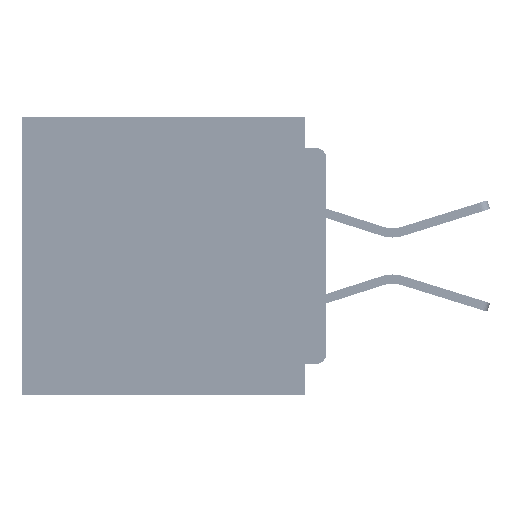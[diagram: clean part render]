
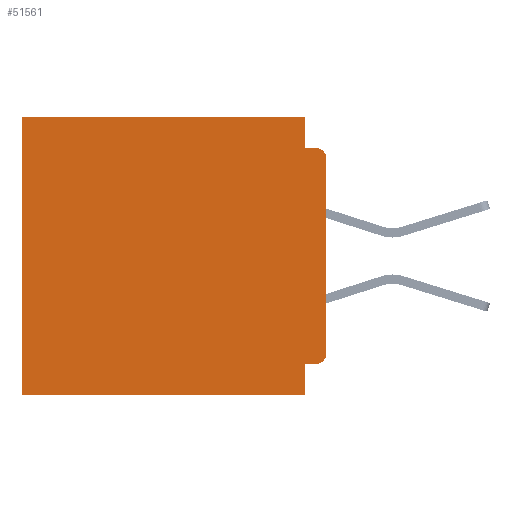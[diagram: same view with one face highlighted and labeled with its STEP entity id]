
A CAD part, left-side view. The second image highlights one B-rep face of the part: STEP entity #51561.
In plain terms, the highlighted planar face has unit normal (-1, 0, 0).
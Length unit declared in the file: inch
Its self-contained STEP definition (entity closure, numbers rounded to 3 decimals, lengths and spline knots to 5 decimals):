
#1955 = ORIENTED_EDGE ( 'NONE', *, *, #10316, .T. ) ;
#1964 = VERTEX_POINT ( 'NONE', #22552 ) ;
#2146 = ORIENTED_EDGE ( 'NONE', *, *, #38919, .F. ) ;
#2992 = CARTESIAN_POINT ( 'NONE',  ( 0.3, 0.031, -0.045 ) ) ;
#3747 = VECTOR ( 'NONE', #14374, 39.37008 ) ;
#8459 = LINE ( 'NONE', #29916, #48163 ) ;
#8708 = LINE ( 'NONE', #55125, #34632 ) ;
#8834 = DIRECTION ( 'NONE',  ( 0., 0., -1. ) ) ;
#9208 = VERTEX_POINT ( 'NONE', #57346 ) ;
#9301 = DIRECTION ( 'NONE',  ( 0., 0., -1. ) ) ;
#10316 = EDGE_CURVE ( 'NONE', #20601, #61688, #58531, .T. ) ;
#10668 = CARTESIAN_POINT ( 'NONE',  ( 0.3, 0.437, -0.4 ) ) ;
#10675 = DIRECTION ( 'NONE',  ( 0., -1., 0. ) ) ;
#10889 = CARTESIAN_POINT ( 'NONE',  ( 0.3, 0.031, 0. ) ) ;
#11165 = CARTESIAN_POINT ( 'NONE',  ( 0.3, 0., -0.355 ) ) ;
#11989 = CARTESIAN_POINT ( 'NONE',  ( 0.3, 0., -0.4 ) ) ;
#12086 = LINE ( 'NONE', #11165, #65411 ) ;
#13186 = DIRECTION ( 'NONE',  ( -1., 0., 0. ) ) ;
#14374 = DIRECTION ( 'NONE',  ( 0., 1., 0. ) ) ;
#15831 = VERTEX_POINT ( 'NONE', #30824 ) ;
#17457 = CIRCLE ( 'NONE', #27039, 0.015 ) ;
#18066 = ORIENTED_EDGE ( 'NONE', *, *, #57772, .T. ) ;
#20601 = VERTEX_POINT ( 'NONE', #36192 ) ;
#20911 = AXIS2_PLACEMENT_3D ( 'NONE', #11989, #63712, #32830 ) ;
#21252 = EDGE_CURVE ( 'NONE', #51878, #15831, #8459, .T. ) ;
#21266 = VECTOR ( 'NONE', #10675, 39.37008 ) ;
#22552 = CARTESIAN_POINT ( 'NONE',  ( 0.3, 0.031, -0.4 ) ) ;
#22602 = ORIENTED_EDGE ( 'NONE', *, *, #51852, .F. ) ;
#24195 = DIRECTION ( 'NONE',  ( 0., 1., 0. ) ) ;
#24232 = FACE_OUTER_BOUND ( 'NONE', #27338, .T. ) ;
#24655 = CARTESIAN_POINT ( 'NONE',  ( 0.3, 0.031, -0.4 ) ) ;
#26128 = EDGE_CURVE ( 'NONE', #46840, #51804, #59398, .T. ) ;
#27039 = AXIS2_PLACEMENT_3D ( 'NONE', #44189, #13186, #49410 ) ;
#27338 = EDGE_LOOP ( 'NONE', ( #35293, #49905, #55408, #66209, #18066, #1955, #50438, #22602, #2146, #40544 ) ) ;
#27469 = CARTESIAN_POINT ( 'NONE',  ( 0.3, 0.015, -0.045 ) ) ;
#27618 = PLANE ( 'NONE',  #20911 ) ;
#28020 = EDGE_CURVE ( 'NONE', #51878, #40833, #51942, .T. ) ;
#29446 = CARTESIAN_POINT ( 'NONE',  ( 0.3, 0.015, -0.06 ) ) ;
#29842 = DIRECTION ( 'NONE',  ( 0., 0., -1. ) ) ;
#29916 = CARTESIAN_POINT ( 'NONE',  ( 0.3, 0., -0.4 ) ) ;
#30824 = CARTESIAN_POINT ( 'NONE',  ( 0.3, 0., -0.34 ) ) ;
#31212 = LINE ( 'NONE', #40145, #3747 ) ;
#31719 = DIRECTION ( 'NONE',  ( 0., 0., -1. ) ) ;
#31785 = AXIS2_PLACEMENT_3D ( 'NONE', #29446, #65534, #34665 ) ;
#32830 = DIRECTION ( 'NONE',  ( 0., 0., -1. ) ) ;
#33904 = VECTOR ( 'NONE', #29842, 39.37008 ) ;
#34632 = VECTOR ( 'NONE', #24195, 39.37008 ) ;
#34665 = DIRECTION ( 'NONE',  ( 0., 0., -1. ) ) ;
#35293 = ORIENTED_EDGE ( 'NONE', *, *, #21252, .F. ) ;
#36192 = CARTESIAN_POINT ( 'NONE',  ( 0.3, 0.437, 0. ) ) ;
#36473 = CARTESIAN_POINT ( 'NONE',  ( 0.3, 0., -0.045 ) ) ;
#38919 = EDGE_CURVE ( 'NONE', #42781, #9208, #12086, .T. ) ;
#39868 = EDGE_CURVE ( 'NONE', #1964, #61688, #8708, .T. ) ;
#40145 = CARTESIAN_POINT ( 'NONE',  ( 0.3, 0., 0. ) ) ;
#40544 = ORIENTED_EDGE ( 'NONE', *, *, #53533, .T. ) ;
#40833 = VERTEX_POINT ( 'NONE', #27469 ) ;
#42781 = VERTEX_POINT ( 'NONE', #54680 ) ;
#44189 = CARTESIAN_POINT ( 'NONE',  ( 0.3, 0.015, -0.34 ) ) ;
#45706 = VECTOR ( 'NONE', #31719, 39.37008 ) ;
#46840 = VERTEX_POINT ( 'NONE', #55636 ) ;
#47668 = LINE ( 'NONE', #24655, #33904 ) ;
#48163 = VECTOR ( 'NONE', #9301, 39.37008 ) ;
#49410 = DIRECTION ( 'NONE',  ( 0., 0., -1. ) ) ;
#49905 = ORIENTED_EDGE ( 'NONE', *, *, #28020, .T. ) ;
#50237 = CARTESIAN_POINT ( 'NONE',  ( 0.3, 0.437, -0.4 ) ) ;
#50400 = LINE ( 'NONE', #36473, #21266 ) ;
#50438 = ORIENTED_EDGE ( 'NONE', *, *, #39868, .F. ) ;
#51561 = ADVANCED_FACE ( 'NONE', ( #24232 ), #27618, .F. ) ;
#51804 = VERTEX_POINT ( 'NONE', #2992 ) ;
#51852 = EDGE_CURVE ( 'NONE', #9208, #1964, #47668, .T. ) ;
#51878 = VERTEX_POINT ( 'NONE', #55581 ) ;
#51942 = CIRCLE ( 'NONE', #31785, 0.015 ) ;
#53533 = EDGE_CURVE ( 'NONE', #42781, #15831, #17457, .T. ) ;
#54680 = CARTESIAN_POINT ( 'NONE',  ( 0.3, 0.015, -0.355 ) ) ;
#55125 = CARTESIAN_POINT ( 'NONE',  ( 0.3, 0., -0.4 ) ) ;
#55408 = ORIENTED_EDGE ( 'NONE', *, *, #63558, .F. ) ;
#55581 = CARTESIAN_POINT ( 'NONE',  ( 0.3, 0., -0.06 ) ) ;
#55636 = CARTESIAN_POINT ( 'NONE',  ( 0.3, 0.031, 0. ) ) ;
#56903 = VECTOR ( 'NONE', #8834, 39.37008 ) ;
#57346 = CARTESIAN_POINT ( 'NONE',  ( 0.3, 0.031, -0.355 ) ) ;
#57717 = DIRECTION ( 'NONE',  ( 0., 1., 0. ) ) ;
#57772 = EDGE_CURVE ( 'NONE', #46840, #20601, #31212, .T. ) ;
#58531 = LINE ( 'NONE', #50237, #56903 ) ;
#59398 = LINE ( 'NONE', #10889, #45706 ) ;
#61688 = VERTEX_POINT ( 'NONE', #10668 ) ;
#63558 = EDGE_CURVE ( 'NONE', #51804, #40833, #50400, .T. ) ;
#63712 = DIRECTION ( 'NONE',  ( 1., 0., 0. ) ) ;
#65411 = VECTOR ( 'NONE', #57717, 39.37008 ) ;
#65534 = DIRECTION ( 'NONE',  ( -1., 0., 0. ) ) ;
#66209 = ORIENTED_EDGE ( 'NONE', *, *, #26128, .F. ) ;
